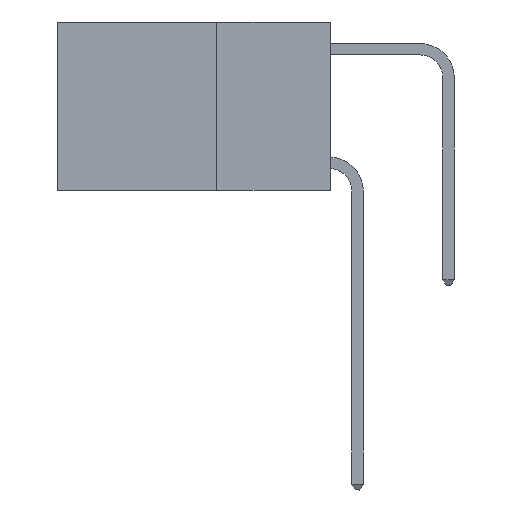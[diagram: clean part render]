
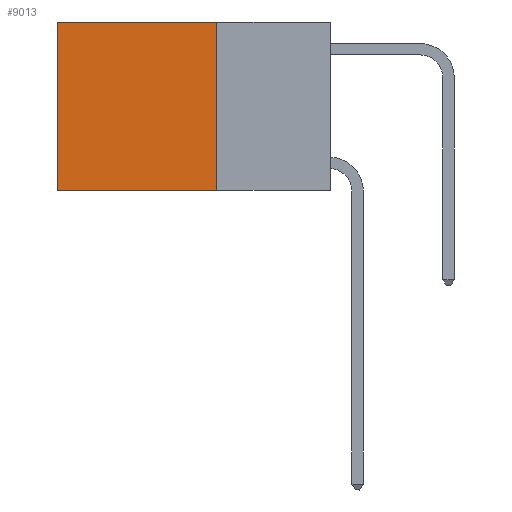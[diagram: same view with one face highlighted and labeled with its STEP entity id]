
A CAD part, left-side view. The second image highlights one B-rep face of the part: STEP entity #9013.
In plain terms, the highlighted planar face has unit normal (-1, 0, 0).
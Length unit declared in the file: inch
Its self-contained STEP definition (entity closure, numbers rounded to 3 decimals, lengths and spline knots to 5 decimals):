
#336 = FACE_OUTER_BOUND ( 'NONE', #4236, .T. ) ;
#723 = VERTEX_POINT ( 'NONE', #8274 ) ;
#729 = DIRECTION ( 'NONE',  ( 0., 0., -1. ) ) ;
#759 = VERTEX_POINT ( 'NONE', #3882 ) ;
#3128 = CARTESIAN_POINT ( 'NONE',  ( 0.2625, 0.25, 0. ) ) ;
#3294 = LINE ( 'NONE', #16022, #10194 ) ;
#3882 = CARTESIAN_POINT ( 'NONE',  ( 0.2625, 0.6, 0. ) ) ;
#4236 = EDGE_LOOP ( 'NONE', ( #10911, #10999, #11117, #11178 ) ) ;
#4376 = CARTESIAN_POINT ( 'NONE',  ( 0.2625, 0.6, -0.37 ) ) ;
#4898 = VECTOR ( 'NONE', #11080, 39.37008 ) ;
#5094 = CARTESIAN_POINT ( 'NONE',  ( 0.2625, 0.6, 0. ) ) ;
#5398 = EDGE_CURVE ( 'NONE', #16760, #723, #8336, .T. ) ;
#5738 = DIRECTION ( 'NONE',  ( 0., 1., 0. ) ) ;
#5802 = VECTOR ( 'NONE', #15116, 39.37008 ) ;
#5930 = CARTESIAN_POINT ( 'NONE',  ( 0.2625, 0.25, 0. ) ) ;
#6127 = CARTESIAN_POINT ( 'NONE',  ( 0.2625, 0.25, 0. ) ) ;
#6968 = EDGE_CURVE ( 'NONE', #759, #9489, #6982, .T. ) ;
#6982 = LINE ( 'NONE', #5094, #9620 ) ;
#7103 = AXIS2_PLACEMENT_3D ( 'NONE', #7276, #8604, #729 ) ;
#7276 = CARTESIAN_POINT ( 'NONE',  ( 0.2625, 0.25, 0. ) ) ;
#8274 = CARTESIAN_POINT ( 'NONE',  ( 0.2625, 0.25, -0.37 ) ) ;
#8336 = LINE ( 'NONE', #5930, #4898 ) ;
#8604 = DIRECTION ( 'NONE',  ( 1., 0., 0. ) ) ;
#9013 = ADVANCED_FACE ( 'NONE', ( #336 ), #16241, .F. ) ;
#9489 = VERTEX_POINT ( 'NONE', #4376 ) ;
#9620 = VECTOR ( 'NONE', #11483, 39.37008 ) ;
#10194 = VECTOR ( 'NONE', #5738, 39.37008 ) ;
#10911 = ORIENTED_EDGE ( 'NONE', *, *, #6968, .T. ) ;
#10999 = ORIENTED_EDGE ( 'NONE', *, *, #15819, .F. ) ;
#11080 = DIRECTION ( 'NONE',  ( 0., 0., -1. ) ) ;
#11117 = ORIENTED_EDGE ( 'NONE', *, *, #5398, .F. ) ;
#11178 = ORIENTED_EDGE ( 'NONE', *, *, #12515, .T. ) ;
#11483 = DIRECTION ( 'NONE',  ( 0., 0., -1. ) ) ;
#12515 = EDGE_CURVE ( 'NONE', #16760, #759, #12629, .T. ) ;
#12629 = LINE ( 'NONE', #6127, #5802 ) ;
#15116 = DIRECTION ( 'NONE',  ( 0., 1., 0. ) ) ;
#15819 = EDGE_CURVE ( 'NONE', #723, #9489, #3294, .T. ) ;
#16022 = CARTESIAN_POINT ( 'NONE',  ( 0.2625, 0.25, -0.37 ) ) ;
#16241 = PLANE ( 'NONE',  #7103 ) ;
#16760 = VERTEX_POINT ( 'NONE', #3128 ) ;
